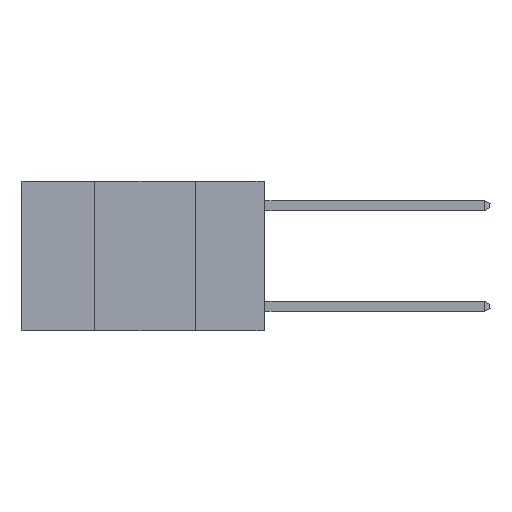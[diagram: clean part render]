
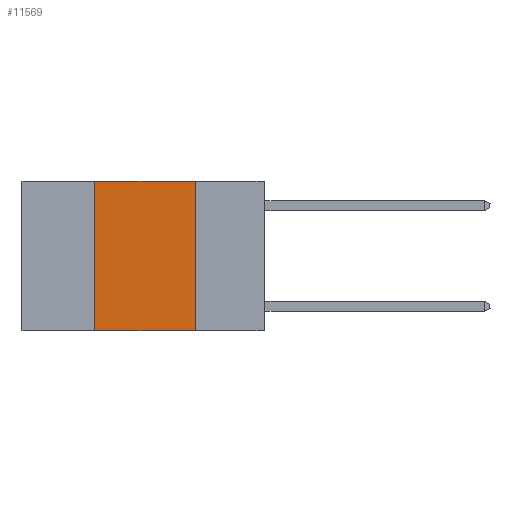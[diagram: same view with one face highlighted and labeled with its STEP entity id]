
A CAD part, left-side view. The second image highlights one B-rep face of the part: STEP entity #11569.
In plain terms, the highlighted planar face has unit normal (-1, 0, 0).
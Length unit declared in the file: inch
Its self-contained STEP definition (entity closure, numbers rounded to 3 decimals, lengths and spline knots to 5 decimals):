
#423 = VERTEX_POINT ( 'NONE', #812 ) ;
#784 = DIRECTION ( 'NONE',  ( 0., 0., 1. ) ) ;
#812 = CARTESIAN_POINT ( 'NONE',  ( 0., 0.17, -0.37 ) ) ;
#1000 = VERTEX_POINT ( 'NONE', #11982 ) ;
#1110 = FACE_OUTER_BOUND ( 'NONE', #3913, .T. ) ;
#1624 = VERTEX_POINT ( 'NONE', #8959 ) ;
#1647 = LINE ( 'NONE', #9207, #7594 ) ;
#1696 = CARTESIAN_POINT ( 'NONE',  ( 0., 0.6, -0.37 ) ) ;
#1767 = ORIENTED_EDGE ( 'NONE', *, *, #6137, .F. ) ;
#2684 = VERTEX_POINT ( 'NONE', #12330 ) ;
#2765 = ORIENTED_EDGE ( 'NONE', *, *, #11673, .F. ) ;
#3805 = LINE ( 'NONE', #1696, #9089 ) ;
#3913 = EDGE_LOOP ( 'NONE', ( #12134, #2765, #1767, #4312 ) ) ;
#3941 = DIRECTION ( 'NONE',  ( 0., -1., 0. ) ) ;
#4312 = ORIENTED_EDGE ( 'NONE', *, *, #7816, .T. ) ;
#4416 = VECTOR ( 'NONE', #784, 39.37008 ) ;
#4513 = AXIS2_PLACEMENT_3D ( 'NONE', #12886, #5425, #13025 ) ;
#5386 = LINE ( 'NONE', #13771, #4416 ) ;
#5425 = DIRECTION ( 'NONE',  ( 1., 0., 0. ) ) ;
#6027 = EDGE_CURVE ( 'NONE', #2684, #423, #1647, .T. ) ;
#6137 = EDGE_CURVE ( 'NONE', #1000, #1624, #5386, .T. ) ;
#6792 = DIRECTION ( 'NONE',  ( 0., -1., 0. ) ) ;
#7594 = VECTOR ( 'NONE', #11418, 39.37008 ) ;
#7816 = EDGE_CURVE ( 'NONE', #1000, #423, #3805, .T. ) ;
#8834 = LINE ( 'NONE', #13168, #11777 ) ;
#8959 = CARTESIAN_POINT ( 'NONE',  ( 0., 0.42, 0. ) ) ;
#9089 = VECTOR ( 'NONE', #3941, 39.37008 ) ;
#9207 = CARTESIAN_POINT ( 'NONE',  ( 0., 0.17, 0. ) ) ;
#11418 = DIRECTION ( 'NONE',  ( 0., 0., -1. ) ) ;
#11569 = ADVANCED_FACE ( 'NONE', ( #1110 ), #11965, .F. ) ;
#11673 = EDGE_CURVE ( 'NONE', #1624, #2684, #8834, .T. ) ;
#11777 = VECTOR ( 'NONE', #6792, 39.37008 ) ;
#11965 = PLANE ( 'NONE',  #4513 ) ;
#11982 = CARTESIAN_POINT ( 'NONE',  ( 0., 0.42, -0.37 ) ) ;
#12134 = ORIENTED_EDGE ( 'NONE', *, *, #6027, .F. ) ;
#12330 = CARTESIAN_POINT ( 'NONE',  ( 0., 0.17, 0. ) ) ;
#12886 = CARTESIAN_POINT ( 'NONE',  ( 0., 0.6, 0. ) ) ;
#13025 = DIRECTION ( 'NONE',  ( 0., 0., -1. ) ) ;
#13168 = CARTESIAN_POINT ( 'NONE',  ( 0., 0.6, 0. ) ) ;
#13771 = CARTESIAN_POINT ( 'NONE',  ( 0., 0.42, 0. ) ) ;
